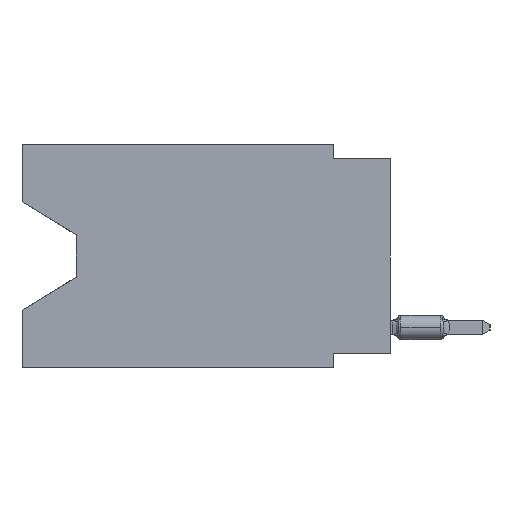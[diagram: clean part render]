
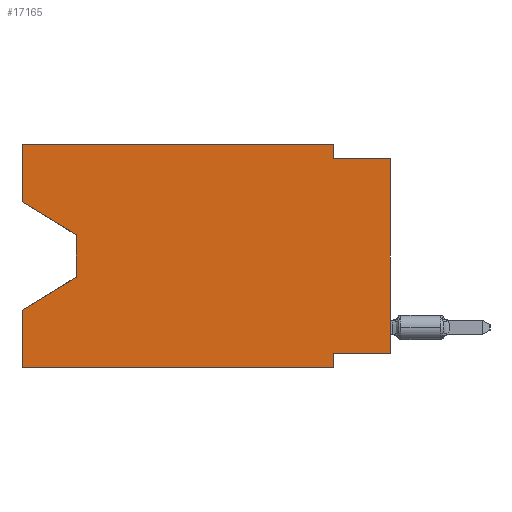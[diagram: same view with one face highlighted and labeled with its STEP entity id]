
A CAD part, left-side view. The second image highlights one B-rep face of the part: STEP entity #17165.
In plain terms, the highlighted planar face has unit normal (-1, 0, 0).
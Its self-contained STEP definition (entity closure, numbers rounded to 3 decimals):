
#255 = VERTEX_POINT ( 'NONE', #3820 ) ;
#438 = PLANE ( 'NONE',  #6281 ) ;
#928 = CARTESIAN_POINT ( 'NONE',  ( 0., 2.54, -0.635 ) ) ;
#1141 = ORIENTED_EDGE ( 'NONE', *, *, #49692, .T. ) ;
#1288 = DIRECTION ( 'NONE',  ( 0., 0., 1. ) ) ;
#1461 = VERTEX_POINT ( 'NONE', #35811 ) ;
#2904 = CARTESIAN_POINT ( 'NONE',  ( 0., 13.97, -5.893 ) ) ;
#3082 = VECTOR ( 'NONE', #43494, 1000. ) ;
#3151 = DIRECTION ( 'NONE',  ( 0., -0.855, -0.519 ) ) ;
#3608 = ORIENTED_EDGE ( 'NONE', *, *, #4169, .T. ) ;
#3763 = LINE ( 'NONE', #60589, #54149 ) ;
#3820 = CARTESIAN_POINT ( 'NONE',  ( 0., 16.383, 0. ) ) ;
#4024 = VECTOR ( 'NONE', #37662, 1000. ) ;
#4169 = EDGE_CURVE ( 'NONE', #57775, #12945, #51495, .T. ) ;
#6281 = AXIS2_PLACEMENT_3D ( 'NONE', #10547, #19761, #46498 ) ;
#6453 = EDGE_CURVE ( 'NONE', #56477, #1461, #8010, .T. ) ;
#6890 = ORIENTED_EDGE ( 'NONE', *, *, #31929, .F. ) ;
#7741 = LINE ( 'NONE', #26486, #57891 ) ;
#8010 = LINE ( 'NONE', #9820, #15030 ) ;
#8122 = ORIENTED_EDGE ( 'NONE', *, *, #12533, .T. ) ;
#9820 = CARTESIAN_POINT ( 'NONE',  ( 0., 2.54, -9.906 ) ) ;
#9828 = VECTOR ( 'NONE', #55955, 1000. ) ;
#10429 = CARTESIAN_POINT ( 'NONE',  ( 0., 0., -9.271 ) ) ;
#10489 = LINE ( 'NONE', #43349, #40494 ) ;
#10547 = CARTESIAN_POINT ( 'NONE',  ( 0., 16.383, 0. ) ) ;
#11153 = VECTOR ( 'NONE', #14761, 1000. ) ;
#12533 = EDGE_CURVE ( 'NONE', #23860, #57775, #25060, .T. ) ;
#12945 = VERTEX_POINT ( 'NONE', #38502 ) ;
#13328 = CARTESIAN_POINT ( 'NONE',  ( 0., 16.383, -9.906 ) ) ;
#14409 = CARTESIAN_POINT ( 'NONE',  ( 0., 16.383, -9.906 ) ) ;
#14419 = DIRECTION ( 'NONE',  ( 0., 0., -1. ) ) ;
#14753 = DIRECTION ( 'NONE',  ( 0., 0., -1. ) ) ;
#14761 = DIRECTION ( 'NONE',  ( 0., -1., 0. ) ) ;
#14840 = EDGE_CURVE ( 'NONE', #27288, #255, #3763, .T. ) ;
#15030 = VECTOR ( 'NONE', #14419, 1000. ) ;
#16935 = DIRECTION ( 'NONE',  ( 0., 0., 1. ) ) ;
#17106 = EDGE_CURVE ( 'NONE', #42645, #1461, #21633, .T. ) ;
#17165 = ADVANCED_FACE ( 'NONE', ( #52632 ), #438, .F. ) ;
#17616 = VECTOR ( 'NONE', #32659, 1000. ) ;
#17938 = DIRECTION ( 'NONE',  ( 0., -1., 0. ) ) ;
#18504 = CARTESIAN_POINT ( 'NONE',  ( 0., 16.383, -2.546 ) ) ;
#18776 = LINE ( 'NONE', #46733, #9828 ) ;
#19357 = LINE ( 'NONE', #28299, #11153 ) ;
#19761 = DIRECTION ( 'NONE',  ( 1., 0., 0. ) ) ;
#19802 = ORIENTED_EDGE ( 'NONE', *, *, #6453, .F. ) ;
#21525 = ORIENTED_EDGE ( 'NONE', *, *, #17106, .T. ) ;
#21633 = LINE ( 'NONE', #13328, #35667 ) ;
#23348 = ORIENTED_EDGE ( 'NONE', *, *, #39709, .F. ) ;
#23860 = VERTEX_POINT ( 'NONE', #30809 ) ;
#24512 = VERTEX_POINT ( 'NONE', #928 ) ;
#24874 = ORIENTED_EDGE ( 'NONE', *, *, #39224, .F. ) ;
#25060 = LINE ( 'NONE', #34846, #3082 ) ;
#25552 = CARTESIAN_POINT ( 'NONE',  ( 0., 16.383, 0. ) ) ;
#26486 = CARTESIAN_POINT ( 'NONE',  ( 0., 16.383, -2.546 ) ) ;
#27288 = VERTEX_POINT ( 'NONE', #18504 ) ;
#28299 = CARTESIAN_POINT ( 'NONE',  ( 0., 16.383, 0. ) ) ;
#28502 = ORIENTED_EDGE ( 'NONE', *, *, #60474, .T. ) ;
#28603 = VERTEX_POINT ( 'NONE', #59526 ) ;
#29100 = VECTOR ( 'NONE', #16935, 1000. ) ;
#30474 = CARTESIAN_POINT ( 'NONE',  ( 0., 2.54, 0. ) ) ;
#30606 = VERTEX_POINT ( 'NONE', #10429 ) ;
#30809 = CARTESIAN_POINT ( 'NONE',  ( 0., 13.97, -4.013 ) ) ;
#31929 = EDGE_CURVE ( 'NONE', #58146, #24512, #56840, .T. ) ;
#32659 = DIRECTION ( 'NONE',  ( 0., 1., 0. ) ) ;
#33091 = EDGE_CURVE ( 'NONE', #255, #58146, #19357, .T. ) ;
#33197 = LINE ( 'NONE', #51418, #17616 ) ;
#34585 = EDGE_CURVE ( 'NONE', #42645, #12945, #54716, .T. ) ;
#34846 = CARTESIAN_POINT ( 'NONE',  ( 0., 13.97, -4.013 ) ) ;
#35667 = VECTOR ( 'NONE', #17938, 1000. ) ;
#35811 = CARTESIAN_POINT ( 'NONE',  ( 0., 2.54, -9.906 ) ) ;
#37662 = DIRECTION ( 'NONE',  ( 0., 0.855, -0.519 ) ) ;
#38502 = CARTESIAN_POINT ( 'NONE',  ( 0., 16.383, -7.36 ) ) ;
#39224 = EDGE_CURVE ( 'NONE', #30606, #56477, #33197, .T. ) ;
#39709 = EDGE_CURVE ( 'NONE', #24512, #28603, #18776, .T. ) ;
#40494 = VECTOR ( 'NONE', #1288, 1000. ) ;
#42455 = ORIENTED_EDGE ( 'NONE', *, *, #34585, .F. ) ;
#42579 = CARTESIAN_POINT ( 'NONE',  ( 0., 13.97, -5.893 ) ) ;
#42645 = VERTEX_POINT ( 'NONE', #14409 ) ;
#43349 = CARTESIAN_POINT ( 'NONE',  ( 0., 0., 0. ) ) ;
#43494 = DIRECTION ( 'NONE',  ( 0., 0., -1. ) ) ;
#46498 = DIRECTION ( 'NONE',  ( 0., 0., -1. ) ) ;
#46733 = CARTESIAN_POINT ( 'NONE',  ( 0., 0., -0.635 ) ) ;
#47034 = ORIENTED_EDGE ( 'NONE', *, *, #14840, .F. ) ;
#49692 = EDGE_CURVE ( 'NONE', #30606, #28603, #10489, .T. ) ;
#50741 = DIRECTION ( 'NONE',  ( 0., 0., 1. ) ) ;
#51418 = CARTESIAN_POINT ( 'NONE',  ( 0., 0., -9.271 ) ) ;
#51495 = LINE ( 'NONE', #42579, #4024 ) ;
#51933 = CARTESIAN_POINT ( 'NONE',  ( 0., 2.54, 0. ) ) ;
#52632 = FACE_OUTER_BOUND ( 'NONE', #52896, .T. ) ;
#52896 = EDGE_LOOP ( 'NONE', ( #28502, #8122, #3608, #42455, #21525, #19802, #24874, #1141, #23348, #6890, #55279, #47034 ) ) ;
#54149 = VECTOR ( 'NONE', #50741, 1000. ) ;
#54257 = VECTOR ( 'NONE', #14753, 1000. ) ;
#54716 = LINE ( 'NONE', #25552, #29100 ) ;
#55279 = ORIENTED_EDGE ( 'NONE', *, *, #33091, .F. ) ;
#55955 = DIRECTION ( 'NONE',  ( 0., -1., 0. ) ) ;
#56477 = VERTEX_POINT ( 'NONE', #58830 ) ;
#56840 = LINE ( 'NONE', #51933, #54257 ) ;
#57775 = VERTEX_POINT ( 'NONE', #2904 ) ;
#57891 = VECTOR ( 'NONE', #3151, 1000. ) ;
#58146 = VERTEX_POINT ( 'NONE', #30474 ) ;
#58830 = CARTESIAN_POINT ( 'NONE',  ( 0., 2.54, -9.271 ) ) ;
#59526 = CARTESIAN_POINT ( 'NONE',  ( 0., 0., -0.635 ) ) ;
#60474 = EDGE_CURVE ( 'NONE', #27288, #23860, #7741, .T. ) ;
#60589 = CARTESIAN_POINT ( 'NONE',  ( 0., 16.383, 0. ) ) ;
